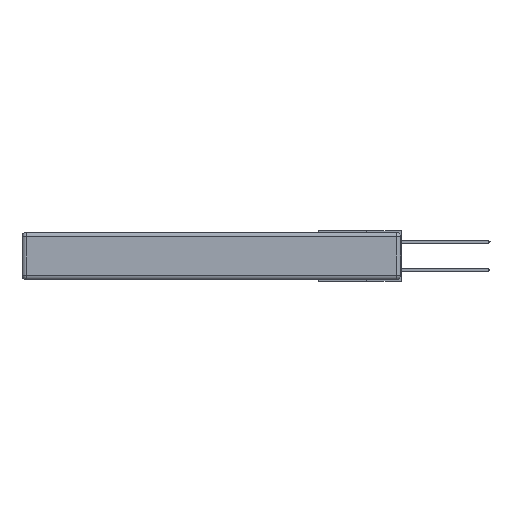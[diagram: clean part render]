
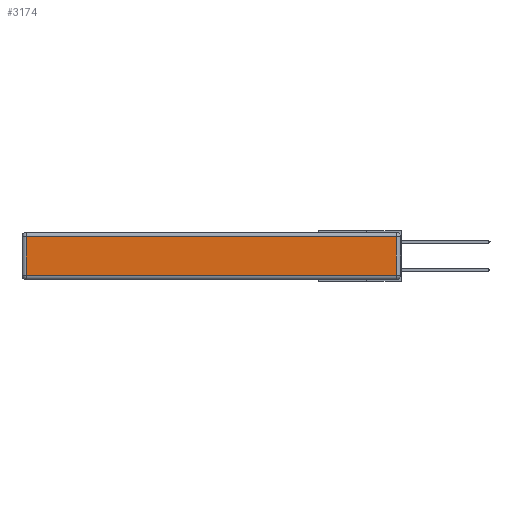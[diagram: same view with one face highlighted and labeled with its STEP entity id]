
A CAD part, left-side view. The second image highlights one B-rep face of the part: STEP entity #3174.
In plain terms, the highlighted planar face has unit normal (-1, 0, 0).
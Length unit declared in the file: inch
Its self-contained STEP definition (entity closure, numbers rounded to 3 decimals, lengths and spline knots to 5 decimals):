
#504 = ORIENTED_EDGE ( 'NONE', *, *, #11993, .T. ) ;
#1226 = DIRECTION ( 'NONE',  ( -1., 0., 0. ) ) ;
#1736 = CARTESIAN_POINT ( 'NONE',  ( 0., 2.72, -0.03 ) ) ;
#3174 = ADVANCED_FACE ( 'NONE', ( #9955 ), #7679, .T. ) ;
#3489 = VECTOR ( 'NONE', #5156, 39.37008 ) ;
#3702 = VERTEX_POINT ( 'NONE', #1736 ) ;
#4090 = CARTESIAN_POINT ( 'NONE',  ( 0., 0., -0.313 ) ) ;
#4262 = EDGE_CURVE ( 'NONE', #5728, #6169, #5274, .T. ) ;
#4293 = LINE ( 'NONE', #4090, #5924 ) ;
#4433 = CARTESIAN_POINT ( 'NONE',  ( 0., 0.03, -0.03 ) ) ;
#5156 = DIRECTION ( 'NONE',  ( 0., 1., 0. ) ) ;
#5274 = LINE ( 'NONE', #8452, #10732 ) ;
#5728 = VERTEX_POINT ( 'NONE', #15051 ) ;
#5924 = VECTOR ( 'NONE', #12016, 39.37008 ) ;
#6169 = VERTEX_POINT ( 'NONE', #4433 ) ;
#6553 = LINE ( 'NONE', #10333, #3489 ) ;
#7679 = PLANE ( 'NONE',  #15500 ) ;
#8452 = CARTESIAN_POINT ( 'NONE',  ( 0., 0.03, -0.343 ) ) ;
#8472 = EDGE_LOOP ( 'NONE', ( #504, #10387, #8705, #10371 ) ) ;
#8705 = ORIENTED_EDGE ( 'NONE', *, *, #15169, .T. ) ;
#9955 = FACE_OUTER_BOUND ( 'NONE', #8472, .T. ) ;
#10246 = DIRECTION ( 'NONE',  ( 0., 0., 1. ) ) ;
#10258 = DIRECTION ( 'NONE',  ( 0., 0., -1. ) ) ;
#10333 = CARTESIAN_POINT ( 'NONE',  ( 0., 2.75, -0.03 ) ) ;
#10371 = ORIENTED_EDGE ( 'NONE', *, *, #11770, .T. ) ;
#10387 = ORIENTED_EDGE ( 'NONE', *, *, #4262, .T. ) ;
#10732 = VECTOR ( 'NONE', #12529, 39.37008 ) ;
#11770 = EDGE_CURVE ( 'NONE', #3702, #15265, #16351, .T. ) ;
#11993 = EDGE_CURVE ( 'NONE', #15265, #5728, #4293, .T. ) ;
#12016 = DIRECTION ( 'NONE',  ( 0., -1., 0. ) ) ;
#12025 = CARTESIAN_POINT ( 'NONE',  ( 0., 2.72, -0.313 ) ) ;
#12529 = DIRECTION ( 'NONE',  ( 0., 0., 1. ) ) ;
#12809 = CARTESIAN_POINT ( 'NONE',  ( 0., 0., -0.343 ) ) ;
#15051 = CARTESIAN_POINT ( 'NONE',  ( 0., 0.03, -0.313 ) ) ;
#15145 = VECTOR ( 'NONE', #10258, 39.37008 ) ;
#15169 = EDGE_CURVE ( 'NONE', #6169, #3702, #6553, .T. ) ;
#15265 = VERTEX_POINT ( 'NONE', #12025 ) ;
#15500 = AXIS2_PLACEMENT_3D ( 'NONE', #12809, #1226, #10246 ) ;
#16351 = LINE ( 'NONE', #16627, #15145 ) ;
#16627 = CARTESIAN_POINT ( 'NONE',  ( 0., 2.72, -0.343 ) ) ;
